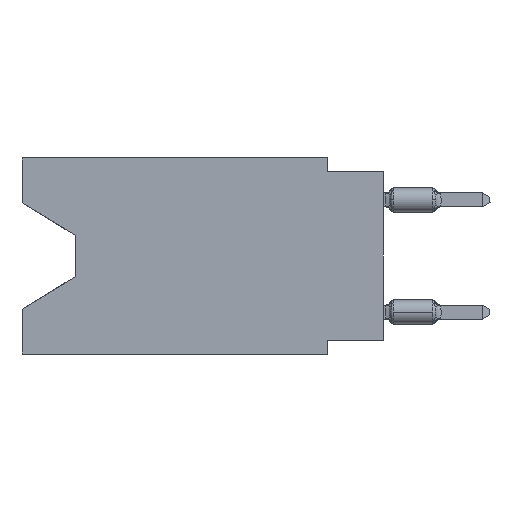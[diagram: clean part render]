
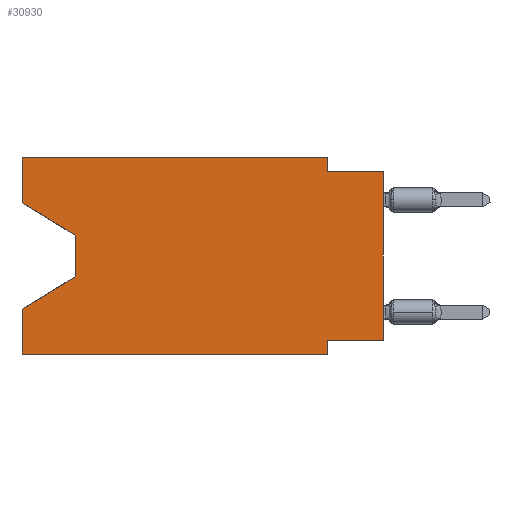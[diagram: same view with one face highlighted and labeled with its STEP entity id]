
A CAD part, left-side view. The second image highlights one B-rep face of the part: STEP entity #30930.
In plain terms, the highlighted planar face has unit normal (-1, 0, 0).
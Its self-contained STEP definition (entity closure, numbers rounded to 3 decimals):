
#329 = VERTEX_POINT ( 'NONE', #17257 ) ;
#1356 = CARTESIAN_POINT ( 'NONE',  ( 0., 16.383, -8.89 ) ) ;
#1420 = VERTEX_POINT ( 'NONE', #30936 ) ;
#1627 = CARTESIAN_POINT ( 'NONE',  ( 0., 2.54, -8.89 ) ) ;
#1650 = AXIS2_PLACEMENT_3D ( 'NONE', #22164, #4919, #29071 ) ;
#1660 = LINE ( 'NONE', #16537, #10114 ) ;
#1777 = CARTESIAN_POINT ( 'NONE',  ( 0., 13.97, -5.385 ) ) ;
#2032 = VECTOR ( 'NONE', #13781, 1000. ) ;
#2234 = CARTESIAN_POINT ( 'NONE',  ( 0., 0., -8.255 ) ) ;
#2428 = CARTESIAN_POINT ( 'NONE',  ( 0., 16.383, -2.038 ) ) ;
#3094 = DIRECTION ( 'NONE',  ( 0., -1., 0. ) ) ;
#3307 = VERTEX_POINT ( 'NONE', #23173 ) ;
#3501 = DIRECTION ( 'NONE',  ( 0., 0., -1. ) ) ;
#3617 = VECTOR ( 'NONE', #3094, 1000. ) ;
#3688 = VERTEX_POINT ( 'NONE', #22301 ) ;
#3990 = ORIENTED_EDGE ( 'NONE', *, *, #4061, .F. ) ;
#4061 = EDGE_CURVE ( 'NONE', #3688, #1420, #13948, .T. ) ;
#4105 = EDGE_CURVE ( 'NONE', #11502, #24841, #10017, .T. ) ;
#4142 = VECTOR ( 'NONE', #23667, 1000. ) ;
#4919 = DIRECTION ( 'NONE',  ( 1., 0., 0. ) ) ;
#5000 = DIRECTION ( 'NONE',  ( 0., -0.855, -0.519 ) ) ;
#5755 = ORIENTED_EDGE ( 'NONE', *, *, #16744, .T. ) ;
#5757 = LINE ( 'NONE', #22372, #3617 ) ;
#6013 = VECTOR ( 'NONE', #3501, 1000. ) ;
#7290 = EDGE_CURVE ( 'NONE', #26655, #11712, #1660, .T. ) ;
#7502 = VERTEX_POINT ( 'NONE', #2234 ) ;
#7920 = EDGE_CURVE ( 'NONE', #7502, #3307, #29969, .T. ) ;
#8184 = VECTOR ( 'NONE', #5000, 1000. ) ;
#8376 = ORIENTED_EDGE ( 'NONE', *, *, #7290, .F. ) ;
#8413 = EDGE_CURVE ( 'NONE', #11712, #17130, #20203, .T. ) ;
#8458 = LINE ( 'NONE', #15820, #17125 ) ;
#9938 = FACE_OUTER_BOUND ( 'NONE', #22911, .T. ) ;
#9997 = LINE ( 'NONE', #17038, #4142 ) ;
#9998 = ORIENTED_EDGE ( 'NONE', *, *, #16290, .F. ) ;
#10017 = LINE ( 'NONE', #28720, #8184 ) ;
#10114 = VECTOR ( 'NONE', #20941, 1000. ) ;
#10687 = DIRECTION ( 'NONE',  ( 0., 0., 1. ) ) ;
#11242 = DIRECTION ( 'NONE',  ( 0., 0., -1. ) ) ;
#11390 = LINE ( 'NONE', #1356, #25599 ) ;
#11502 = VERTEX_POINT ( 'NONE', #2428 ) ;
#11562 = VECTOR ( 'NONE', #11242, 1000. ) ;
#11712 = VERTEX_POINT ( 'NONE', #28217 ) ;
#13016 = CARTESIAN_POINT ( 'NONE',  ( 0., 2.54, -8.89 ) ) ;
#13376 = LINE ( 'NONE', #1627, #6013 ) ;
#13781 = DIRECTION ( 'NONE',  ( 0., 0.855, -0.519 ) ) ;
#13948 = LINE ( 'NONE', #16457, #21218 ) ;
#14114 = DIRECTION ( 'NONE',  ( 0., 0., 1. ) ) ;
#14359 = ORIENTED_EDGE ( 'NONE', *, *, #23260, .F. ) ;
#15514 = CARTESIAN_POINT ( 'NONE',  ( 0., 0., 0. ) ) ;
#15643 = EDGE_CURVE ( 'NONE', #7502, #329, #9997, .T. ) ;
#15776 = EDGE_CURVE ( 'NONE', #17130, #3307, #5757, .T. ) ;
#15787 = ORIENTED_EDGE ( 'NONE', *, *, #4105, .T. ) ;
#15805 = CARTESIAN_POINT ( 'NONE',  ( 0., 16.383, 0. ) ) ;
#15820 = CARTESIAN_POINT ( 'NONE',  ( 0., 16.383, 0. ) ) ;
#16290 = EDGE_CURVE ( 'NONE', #329, #27355, #13376, .T. ) ;
#16457 = CARTESIAN_POINT ( 'NONE',  ( 0., 16.383, 0. ) ) ;
#16537 = CARTESIAN_POINT ( 'NONE',  ( 0., 16.383, 0. ) ) ;
#16744 = EDGE_CURVE ( 'NONE', #29510, #1420, #23673, .T. ) ;
#16892 = ORIENTED_EDGE ( 'NONE', *, *, #15643, .F. ) ;
#17038 = CARTESIAN_POINT ( 'NONE',  ( 0., 0., -8.255 ) ) ;
#17125 = VECTOR ( 'NONE', #18183, 1000. ) ;
#17130 = VERTEX_POINT ( 'NONE', #25356 ) ;
#17143 = EDGE_CURVE ( 'NONE', #3688, #27355, #11390, .T. ) ;
#17172 = ORIENTED_EDGE ( 'NONE', *, *, #20129, .T. ) ;
#17257 = CARTESIAN_POINT ( 'NONE',  ( 0., 2.54, -8.255 ) ) ;
#17982 = DIRECTION ( 'NONE',  ( 0., 0., -1. ) ) ;
#18183 = DIRECTION ( 'NONE',  ( 0., 0., 1. ) ) ;
#18915 = CARTESIAN_POINT ( 'NONE',  ( 0., 13.97, -3.505 ) ) ;
#19051 = VECTOR ( 'NONE', #17982, 1000. ) ;
#19473 = ORIENTED_EDGE ( 'NONE', *, *, #17143, .T. ) ;
#20129 = EDGE_CURVE ( 'NONE', #24841, #29510, #20806, .T. ) ;
#20203 = LINE ( 'NONE', #27275, #19051 ) ;
#20377 = ORIENTED_EDGE ( 'NONE', *, *, #8413, .F. ) ;
#20574 = VECTOR ( 'NONE', #10687, 1000. ) ;
#20806 = LINE ( 'NONE', #18915, #11562 ) ;
#20941 = DIRECTION ( 'NONE',  ( 0., -1., 0. ) ) ;
#21218 = VECTOR ( 'NONE', #14114, 1000. ) ;
#21626 = CARTESIAN_POINT ( 'NONE',  ( 0., 13.97, -3.505 ) ) ;
#22164 = CARTESIAN_POINT ( 'NONE',  ( 0., 16.383, 0. ) ) ;
#22301 = CARTESIAN_POINT ( 'NONE',  ( 0., 16.383, -8.89 ) ) ;
#22372 = CARTESIAN_POINT ( 'NONE',  ( 0., 0., -0.635 ) ) ;
#22844 = DIRECTION ( 'NONE',  ( 0., -1., 0. ) ) ;
#22911 = EDGE_LOOP ( 'NONE', ( #15787, #17172, #5755, #3990, #19473, #9998, #16892, #27588, #26014, #20377, #8376, #14359 ) ) ;
#23173 = CARTESIAN_POINT ( 'NONE',  ( 0., 0., -0.635 ) ) ;
#23203 = CARTESIAN_POINT ( 'NONE',  ( 0., 13.97, -5.385 ) ) ;
#23260 = EDGE_CURVE ( 'NONE', #11502, #26655, #8458, .T. ) ;
#23667 = DIRECTION ( 'NONE',  ( 0., 1., 0. ) ) ;
#23673 = LINE ( 'NONE', #23203, #2032 ) ;
#24841 = VERTEX_POINT ( 'NONE', #21626 ) ;
#25356 = CARTESIAN_POINT ( 'NONE',  ( 0., 2.54, -0.635 ) ) ;
#25599 = VECTOR ( 'NONE', #22844, 1000. ) ;
#26014 = ORIENTED_EDGE ( 'NONE', *, *, #15776, .F. ) ;
#26410 = PLANE ( 'NONE',  #1650 ) ;
#26655 = VERTEX_POINT ( 'NONE', #15805 ) ;
#27275 = CARTESIAN_POINT ( 'NONE',  ( 0., 2.54, 0. ) ) ;
#27355 = VERTEX_POINT ( 'NONE', #13016 ) ;
#27588 = ORIENTED_EDGE ( 'NONE', *, *, #7920, .T. ) ;
#28217 = CARTESIAN_POINT ( 'NONE',  ( 0., 2.54, 0. ) ) ;
#28720 = CARTESIAN_POINT ( 'NONE',  ( 0., 16.383, -2.038 ) ) ;
#29071 = DIRECTION ( 'NONE',  ( 0., 0., -1. ) ) ;
#29510 = VERTEX_POINT ( 'NONE', #1777 ) ;
#29969 = LINE ( 'NONE', #15514, #20574 ) ;
#30930 = ADVANCED_FACE ( 'NONE', ( #9938 ), #26410, .F. ) ;
#30936 = CARTESIAN_POINT ( 'NONE',  ( 0., 16.383, -6.852 ) ) ;
